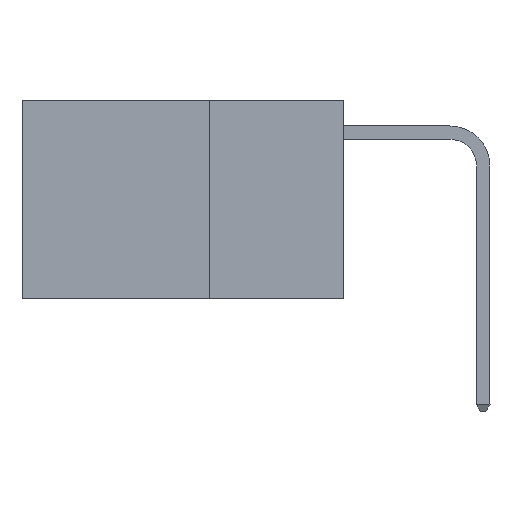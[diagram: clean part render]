
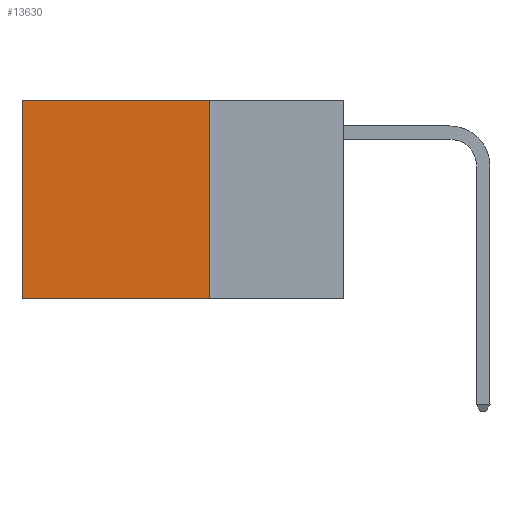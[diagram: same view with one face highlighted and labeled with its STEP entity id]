
A CAD part, left-side view. The second image highlights one B-rep face of the part: STEP entity #13630.
In plain terms, the highlighted planar face has unit normal (-1, 0, 0).
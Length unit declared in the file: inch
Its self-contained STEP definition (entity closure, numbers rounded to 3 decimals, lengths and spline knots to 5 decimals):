
#38 = DIRECTION ( 'NONE',  ( 1., 0., 0. ) ) ;
#163 = ORIENTED_EDGE ( 'NONE', *, *, #2332, .T. ) ;
#690 = LINE ( 'NONE', #16278, #2263 ) ;
#2263 = VECTOR ( 'NONE', #13521, 39.37008 ) ;
#2332 = EDGE_CURVE ( 'NONE', #2955, #8818, #690, .T. ) ;
#2790 = FACE_OUTER_BOUND ( 'NONE', #6654, .T. ) ;
#2955 = VERTEX_POINT ( 'NONE', #3980 ) ;
#3461 = LINE ( 'NONE', #16190, #11351 ) ;
#3980 = CARTESIAN_POINT ( 'NONE',  ( 0.2625, 0.25, 0. ) ) ;
#4849 = DIRECTION ( 'NONE',  ( 0., 1., 0. ) ) ;
#5874 = CARTESIAN_POINT ( 'NONE',  ( 0.2625, 0.6, 0. ) ) ;
#6498 = LINE ( 'NONE', #11981, #8689 ) ;
#6557 = EDGE_CURVE ( 'NONE', #8818, #18026, #13111, .T. ) ;
#6654 = EDGE_LOOP ( 'NONE', ( #11652, #14591, #8838, #163 ) ) ;
#6792 = AXIS2_PLACEMENT_3D ( 'NONE', #15254, #38, #9828 ) ;
#7203 = EDGE_CURVE ( 'NONE', #17085, #18026, #6498, .T. ) ;
#7606 = EDGE_CURVE ( 'NONE', #2955, #17085, #3461, .T. ) ;
#8353 = PLANE ( 'NONE',  #6792 ) ;
#8689 = VECTOR ( 'NONE', #4849, 39.37008 ) ;
#8818 = VERTEX_POINT ( 'NONE', #11510 ) ;
#8838 = ORIENTED_EDGE ( 'NONE', *, *, #7606, .F. ) ;
#9828 = DIRECTION ( 'NONE',  ( 0., 0., -1. ) ) ;
#11351 = VECTOR ( 'NONE', #14816, 39.37008 ) ;
#11510 = CARTESIAN_POINT ( 'NONE',  ( 0.2625, 0.6, 0. ) ) ;
#11652 = ORIENTED_EDGE ( 'NONE', *, *, #6557, .T. ) ;
#11921 = CARTESIAN_POINT ( 'NONE',  ( 0.2625, 0.6, -0.37 ) ) ;
#11981 = CARTESIAN_POINT ( 'NONE',  ( 0.2625, 0.25, -0.37 ) ) ;
#13111 = LINE ( 'NONE', #5874, #14561 ) ;
#13521 = DIRECTION ( 'NONE',  ( 0., 1., 0. ) ) ;
#13630 = ADVANCED_FACE ( 'NONE', ( #2790 ), #8353, .F. ) ;
#14396 = DIRECTION ( 'NONE',  ( 0., 0., -1. ) ) ;
#14561 = VECTOR ( 'NONE', #14396, 39.37008 ) ;
#14591 = ORIENTED_EDGE ( 'NONE', *, *, #7203, .F. ) ;
#14816 = DIRECTION ( 'NONE',  ( 0., 0., -1. ) ) ;
#15043 = CARTESIAN_POINT ( 'NONE',  ( 0.2625, 0.25, -0.37 ) ) ;
#15254 = CARTESIAN_POINT ( 'NONE',  ( 0.2625, 0.25, 0. ) ) ;
#16190 = CARTESIAN_POINT ( 'NONE',  ( 0.2625, 0.25, 0. ) ) ;
#16278 = CARTESIAN_POINT ( 'NONE',  ( 0.2625, 0.25, 0. ) ) ;
#17085 = VERTEX_POINT ( 'NONE', #15043 ) ;
#18026 = VERTEX_POINT ( 'NONE', #11921 ) ;
